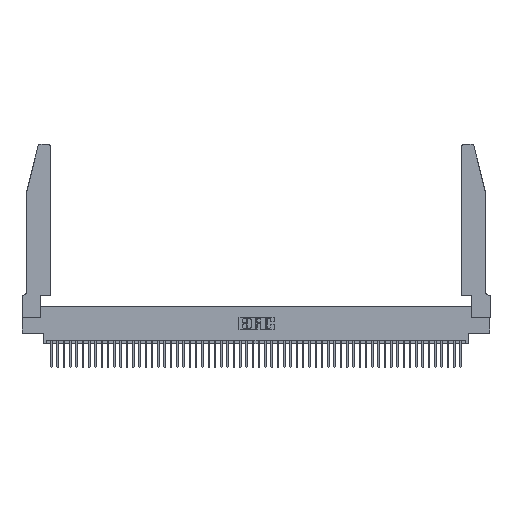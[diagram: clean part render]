
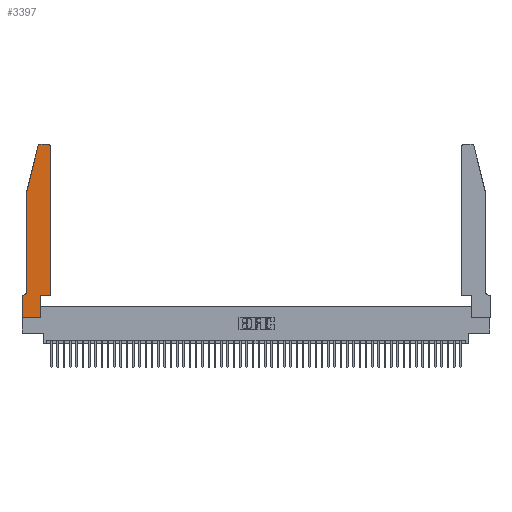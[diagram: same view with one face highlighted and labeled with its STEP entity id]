
A CAD part, top view. The second image highlights one B-rep face of the part: STEP entity #3397.
In plain terms, the highlighted planar face has unit normal (0, 0, 1).
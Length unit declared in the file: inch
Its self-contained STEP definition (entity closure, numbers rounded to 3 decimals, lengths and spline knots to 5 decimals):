
#1136 = EDGE_CURVE ( 'NONE', #2287, #42293, #40447, .T. ) ;
#1500 = DIRECTION ( 'NONE',  ( 0., 0., 1. ) ) ;
#1539 = CARTESIAN_POINT ( 'NONE',  ( 0.2865, 0.35, 0.37 ) ) ;
#1773 = CARTESIAN_POINT ( 'NONE',  ( 0.25487, 2.72718, 0.37 ) ) ;
#1780 = ORIENTED_EDGE ( 'NONE', *, *, #34971, .T. ) ;
#2287 = VERTEX_POINT ( 'NONE', #23371 ) ;
#2531 = VECTOR ( 'NONE', #4832, 39.37008 ) ;
#3397 = ADVANCED_FACE ( 'NONE', ( #41482 ), #26318, .T. ) ;
#3811 = EDGE_CURVE ( 'NONE', #51452, #2287, #44005, .T. ) ;
#3816 = VECTOR ( 'NONE', #52266, 39.37008 ) ;
#4160 = DIRECTION ( 'NONE',  ( 0., 0., 1. ) ) ;
#4800 = VECTOR ( 'NONE', #49279, 39.37008 ) ;
#4832 = DIRECTION ( 'NONE',  ( -1., 0., 0. ) ) ;
#6950 = AXIS2_PLACEMENT_3D ( 'NONE', #13897, #1500, #30465 ) ;
#7266 = VECTOR ( 'NONE', #22224, 39.37008 ) ;
#7835 = ORIENTED_EDGE ( 'NONE', *, *, #11649, .T. ) ;
#7855 = EDGE_LOOP ( 'NONE', ( #9622, #7835, #51336, #8671, #27765, #37965, #40095, #1780, #41205, #12905, #14771, #8269 ) ) ;
#7980 = VERTEX_POINT ( 'NONE', #12117 ) ;
#8269 = ORIENTED_EDGE ( 'NONE', *, *, #31020, .T. ) ;
#8671 = ORIENTED_EDGE ( 'NONE', *, *, #1136, .T. ) ;
#9091 = EDGE_CURVE ( 'NONE', #42293, #7980, #44062, .T. ) ;
#9132 = VERTEX_POINT ( 'NONE', #35864 ) ;
#9589 = DIRECTION ( 'NONE',  ( 0., 0., 1. ) ) ;
#9622 = ORIENTED_EDGE ( 'NONE', *, *, #51867, .T. ) ;
#9941 = VERTEX_POINT ( 'NONE', #49189 ) ;
#11514 = CIRCLE ( 'NONE', #31140, 0.03 ) ;
#11649 = EDGE_CURVE ( 'NONE', #51700, #51452, #11514, .T. ) ;
#11994 = EDGE_CURVE ( 'NONE', #7980, #19664, #28926, .T. ) ;
#12117 = CARTESIAN_POINT ( 'NONE',  ( 0.0055, 0.35, 0.37 ) ) ;
#12905 = ORIENTED_EDGE ( 'NONE', *, *, #30625, .T. ) ;
#13010 = CARTESIAN_POINT ( 'NONE',  ( 0.2605, 2.75, 0.37 ) ) ;
#13713 = AXIS2_PLACEMENT_3D ( 'NONE', #14935, #43745, #19096 ) ;
#13897 = CARTESIAN_POINT ( 'NONE',  ( 0., 0.35, 0.37 ) ) ;
#14060 = CARTESIAN_POINT ( 'NONE',  ( 0.4505, 0.35, 0.37 ) ) ;
#14771 = ORIENTED_EDGE ( 'NONE', *, *, #39973, .T. ) ;
#14935 = CARTESIAN_POINT ( 'NONE',  ( 0.0055, 0.42, 0.37 ) ) ;
#15064 = CARTESIAN_POINT ( 'NONE',  ( 0.0755, 0.42, 0.37 ) ) ;
#16366 = CARTESIAN_POINT ( 'NONE',  ( 0.0755, 2., 0.37 ) ) ;
#18304 = LINE ( 'NONE', #1539, #7266 ) ;
#18464 = VECTOR ( 'NONE', #51362, 39.37008 ) ;
#18532 = VECTOR ( 'NONE', #26366, 39.37008 ) ;
#18541 = VECTOR ( 'NONE', #19001, 39.37008 ) ;
#19001 = DIRECTION ( 'NONE',  ( 1., 0., 0. ) ) ;
#19020 = CARTESIAN_POINT ( 'NONE',  ( 0.0755, 0.35, 0.37 ) ) ;
#19096 = DIRECTION ( 'NONE',  ( -1., 0., 0. ) ) ;
#19386 = VERTEX_POINT ( 'NONE', #27785 ) ;
#19550 = CARTESIAN_POINT ( 'NONE',  ( 0.2865, 0.35, 0.37 ) ) ;
#19603 = CARTESIAN_POINT ( 'NONE',  ( 0.4505, 0.35, 0.37 ) ) ;
#19664 = VERTEX_POINT ( 'NONE', #29972 ) ;
#19763 = LINE ( 'NONE', #47220, #18464 ) ;
#21048 = VECTOR ( 'NONE', #44259, 39.37008 ) ;
#22224 = DIRECTION ( 'NONE',  ( 0., 1., 0. ) ) ;
#22327 = LINE ( 'NONE', #19603, #21048 ) ;
#23371 = CARTESIAN_POINT ( 'NONE',  ( 0.0755, 2., 0.37 ) ) ;
#24592 = LINE ( 'NONE', #13010, #2531 ) ;
#26318 = PLANE ( 'NONE',  #6950 ) ;
#26366 = DIRECTION ( 'NONE',  ( 0., -1., 0. ) ) ;
#27765 = ORIENTED_EDGE ( 'NONE', *, *, #9091, .T. ) ;
#27785 = CARTESIAN_POINT ( 'NONE',  ( 0.4205, 2.75, 0.37 ) ) ;
#28926 = LINE ( 'NONE', #19020, #50780 ) ;
#28948 = CARTESIAN_POINT ( 'NONE',  ( 0.284, 2.72, 0.37 ) ) ;
#29972 = CARTESIAN_POINT ( 'NONE',  ( 0., 0.35, 0.37 ) ) ;
#30465 = DIRECTION ( 'NONE',  ( 1., 0., 0. ) ) ;
#30625 = EDGE_CURVE ( 'NONE', #46360, #40637, #22327, .T. ) ;
#31020 = EDGE_CURVE ( 'NONE', #9941, #19386, #35852, .T. ) ;
#31140 = AXIS2_PLACEMENT_3D ( 'NONE', #28948, #4160, #33129 ) ;
#33129 = DIRECTION ( 'NONE',  ( 1., 0., 0. ) ) ;
#34358 = CARTESIAN_POINT ( 'NONE',  ( 0.4205, 2.72, 0.37 ) ) ;
#34870 = CARTESIAN_POINT ( 'NONE',  ( 0.0755, 2., 0.37 ) ) ;
#34971 = EDGE_CURVE ( 'NONE', #35222, #9132, #50050, .T. ) ;
#35222 = VERTEX_POINT ( 'NONE', #45043 ) ;
#35434 = DIRECTION ( 'NONE',  ( -1., 0., 0. ) ) ;
#35852 = CIRCLE ( 'NONE', #43901, 0.03 ) ;
#35864 = CARTESIAN_POINT ( 'NONE',  ( 0.2865, 0., 0.37 ) ) ;
#35947 = CARTESIAN_POINT ( 'NONE',  ( 0., 0., 0.37 ) ) ;
#36814 = LINE ( 'NONE', #35947, #3816 ) ;
#37962 = EDGE_CURVE ( 'NONE', #9132, #46360, #18304, .T. ) ;
#37965 = ORIENTED_EDGE ( 'NONE', *, *, #11994, .T. ) ;
#38470 = DIRECTION ( 'NONE',  ( 1., 0., 0. ) ) ;
#39973 = EDGE_CURVE ( 'NONE', #40637, #9941, #19763, .T. ) ;
#40095 = ORIENTED_EDGE ( 'NONE', *, *, #47788, .T. ) ;
#40447 = LINE ( 'NONE', #34870, #18532 ) ;
#40637 = VERTEX_POINT ( 'NONE', #14060 ) ;
#41205 = ORIENTED_EDGE ( 'NONE', *, *, #37962, .T. ) ;
#41482 = FACE_OUTER_BOUND ( 'NONE', #7855, .T. ) ;
#42293 = VERTEX_POINT ( 'NONE', #15064 ) ;
#43643 = CARTESIAN_POINT ( 'NONE',  ( 0., 0., 0.37 ) ) ;
#43745 = DIRECTION ( 'NONE',  ( 0., 0., -1. ) ) ;
#43901 = AXIS2_PLACEMENT_3D ( 'NONE', #34358, #9589, #38470 ) ;
#44005 = LINE ( 'NONE', #16366, #4800 ) ;
#44062 = CIRCLE ( 'NONE', #13713, 0.07 ) ;
#44259 = DIRECTION ( 'NONE',  ( 1., 0., 0. ) ) ;
#45043 = CARTESIAN_POINT ( 'NONE',  ( 0., 0., 0.37 ) ) ;
#46360 = VERTEX_POINT ( 'NONE', #19550 ) ;
#47220 = CARTESIAN_POINT ( 'NONE',  ( 0.4505, 0.35, 0.37 ) ) ;
#47788 = EDGE_CURVE ( 'NONE', #19664, #35222, #36814, .T. ) ;
#49189 = CARTESIAN_POINT ( 'NONE',  ( 0.4505, 2.72, 0.37 ) ) ;
#49279 = DIRECTION ( 'NONE',  ( -0.239, -0.971, 0. ) ) ;
#50050 = LINE ( 'NONE', #43643, #18541 ) ;
#50780 = VECTOR ( 'NONE', #35434, 39.37008 ) ;
#51336 = ORIENTED_EDGE ( 'NONE', *, *, #3811, .T. ) ;
#51362 = DIRECTION ( 'NONE',  ( 0., 1., 0. ) ) ;
#51452 = VERTEX_POINT ( 'NONE', #1773 ) ;
#51700 = VERTEX_POINT ( 'NONE', #52814 ) ;
#51867 = EDGE_CURVE ( 'NONE', #19386, #51700, #24592, .T. ) ;
#52266 = DIRECTION ( 'NONE',  ( 0., -1., 0. ) ) ;
#52814 = CARTESIAN_POINT ( 'NONE',  ( 0.284, 2.75, 0.37 ) ) ;
